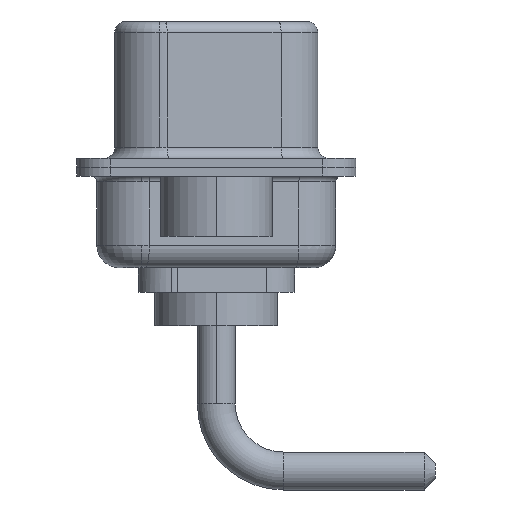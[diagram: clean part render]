
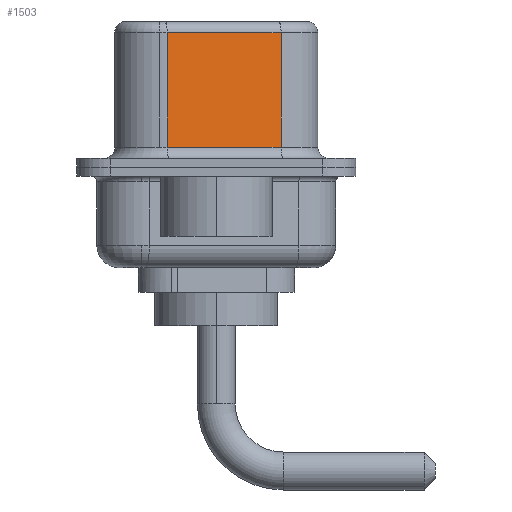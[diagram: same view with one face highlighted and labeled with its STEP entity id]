
A CAD part, left-side view. The second image highlights one B-rep face of the part: STEP entity #1503.
In plain terms, the highlighted planar face has unit normal (-0.985, -0.174, 0).
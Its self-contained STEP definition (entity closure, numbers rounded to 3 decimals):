
#378 = VECTOR ( 'NONE', #965, 1000. ) ;
#965 = DIRECTION ( 'NONE',  ( -0.174, 0.985, 0. ) ) ;
#1274 = ORIENTED_EDGE ( 'NONE', *, *, #14357, .F. ) ;
#1503 = ADVANCED_FACE ( 'NONE', ( #2998 ), #12423, .F. ) ;
#1559 = LINE ( 'NONE', #13755, #12672 ) ;
#2481 = EDGE_CURVE ( 'NONE', #5592, #9664, #12128, .T. ) ;
#2998 = FACE_OUTER_BOUND ( 'NONE', #3507, .T. ) ;
#3291 = DIRECTION ( 'NONE',  ( -0.174, 0.985, 0. ) ) ;
#3425 = DIRECTION ( 'NONE',  ( 0.174, -0.985, 0. ) ) ;
#3507 = EDGE_LOOP ( 'NONE', ( #1274, #5986, #9428, #12237 ) ) ;
#4100 = CARTESIAN_POINT ( 'NONE',  ( 4.58, -2.897, 6.02 ) ) ;
#5466 = DIRECTION ( 'NONE',  ( 0.985, 0.174, 0. ) ) ;
#5579 = CARTESIAN_POINT ( 'NONE',  ( 3.68, 2.203, 0.9 ) ) ;
#5592 = VERTEX_POINT ( 'NONE', #6721 ) ;
#5986 = ORIENTED_EDGE ( 'NONE', *, *, #2481, .T. ) ;
#6010 = VERTEX_POINT ( 'NONE', #10831 ) ;
#6106 = CARTESIAN_POINT ( 'NONE',  ( 3.68, 2.203, 6.52 ) ) ;
#6721 = CARTESIAN_POINT ( 'NONE',  ( 4.58, -2.897, 6.02 ) ) ;
#7102 = DIRECTION ( 'NONE',  ( 0., 0., -1. ) ) ;
#7507 = VECTOR ( 'NONE', #3425, 1000. ) ;
#9428 = ORIENTED_EDGE ( 'NONE', *, *, #11124, .T. ) ;
#9478 = VERTEX_POINT ( 'NONE', #5579 ) ;
#9664 = VERTEX_POINT ( 'NONE', #11447 ) ;
#10564 = DIRECTION ( 'NONE',  ( 0., 0., -1. ) ) ;
#10831 = CARTESIAN_POINT ( 'NONE',  ( 4.58, -2.897, 0.9 ) ) ;
#11124 = EDGE_CURVE ( 'NONE', #9664, #9478, #13720, .T. ) ;
#11182 = CARTESIAN_POINT ( 'NONE',  ( 4.58, -2.897, 6.52 ) ) ;
#11447 = CARTESIAN_POINT ( 'NONE',  ( 3.68, 2.203, 6.02 ) ) ;
#12128 = LINE ( 'NONE', #4100, #378 ) ;
#12237 = ORIENTED_EDGE ( 'NONE', *, *, #13982, .T. ) ;
#12423 = PLANE ( 'NONE',  #12695 ) ;
#12672 = VECTOR ( 'NONE', #7102, 1000. ) ;
#12695 = AXIS2_PLACEMENT_3D ( 'NONE', #11182, #5466, #3291 ) ;
#12812 = VECTOR ( 'NONE', #10564, 1000. ) ;
#12937 = CARTESIAN_POINT ( 'NONE',  ( 4.58, -2.897, 0.9 ) ) ;
#13720 = LINE ( 'NONE', #6106, #12812 ) ;
#13755 = CARTESIAN_POINT ( 'NONE',  ( 4.58, -2.897, 6.52 ) ) ;
#13982 = EDGE_CURVE ( 'NONE', #9478, #6010, #14251, .T. ) ;
#14251 = LINE ( 'NONE', #12937, #7507 ) ;
#14357 = EDGE_CURVE ( 'NONE', #5592, #6010, #1559, .T. ) ;
